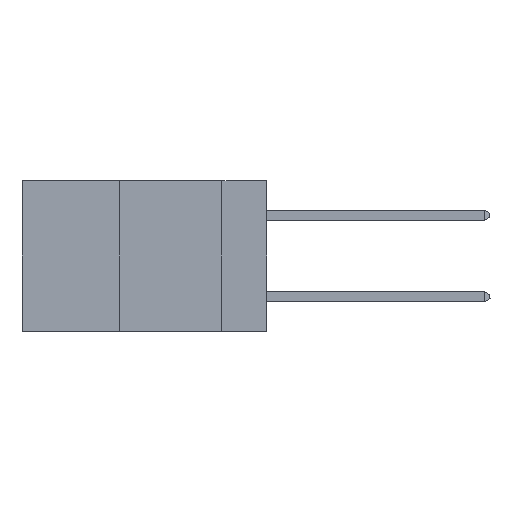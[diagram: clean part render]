
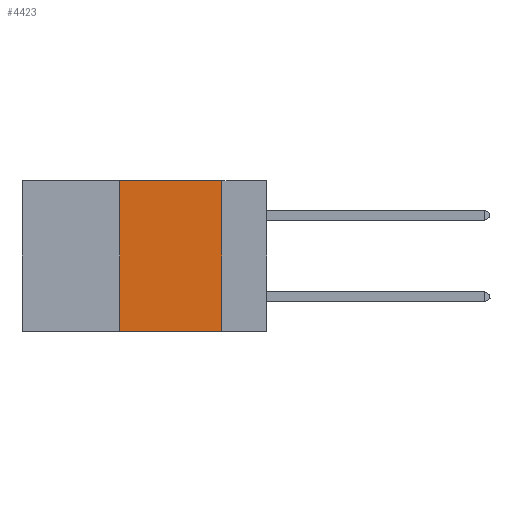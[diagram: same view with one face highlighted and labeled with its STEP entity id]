
A CAD part, left-side view. The second image highlights one B-rep face of the part: STEP entity #4423.
In plain terms, the highlighted planar face has unit normal (-1, 0, 0).
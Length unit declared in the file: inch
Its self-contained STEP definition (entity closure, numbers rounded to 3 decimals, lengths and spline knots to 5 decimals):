
#559 = CARTESIAN_POINT ( 'NONE',  ( 0., 0.36, -0.37 ) ) ;
#588 = EDGE_CURVE ( 'NONE', #12321, #1417, #3090, .T. ) ;
#690 = DIRECTION ( 'NONE',  ( 0., 0., -1. ) ) ;
#1274 = ORIENTED_EDGE ( 'NONE', *, *, #3886, .F. ) ;
#1417 = VERTEX_POINT ( 'NONE', #10688 ) ;
#1654 = VECTOR ( 'NONE', #15829, 39.37008 ) ;
#2398 = CARTESIAN_POINT ( 'NONE',  ( 0., 0.6, -0.37 ) ) ;
#2725 = ORIENTED_EDGE ( 'NONE', *, *, #12848, .F. ) ;
#2737 = VERTEX_POINT ( 'NONE', #11798 ) ;
#3090 = LINE ( 'NONE', #2398, #12622 ) ;
#3165 = ORIENTED_EDGE ( 'NONE', *, *, #588, .T. ) ;
#3886 = EDGE_CURVE ( 'NONE', #7352, #1417, #9478, .T. ) ;
#4423 = ADVANCED_FACE ( 'NONE', ( #5121 ), #16276, .F. ) ;
#5121 = FACE_OUTER_BOUND ( 'NONE', #7189, .T. ) ;
#7189 = EDGE_LOOP ( 'NONE', ( #1274, #9500, #2725, #3165 ) ) ;
#7352 = VERTEX_POINT ( 'NONE', #15607 ) ;
#7427 = LINE ( 'NONE', #10276, #13928 ) ;
#8533 = DIRECTION ( 'NONE',  ( 1., 0., 0. ) ) ;
#9025 = LINE ( 'NONE', #14522, #1654 ) ;
#9478 = LINE ( 'NONE', #13418, #15942 ) ;
#9500 = ORIENTED_EDGE ( 'NONE', *, *, #10750, .F. ) ;
#10276 = CARTESIAN_POINT ( 'NONE',  ( 0., 0.6, 0. ) ) ;
#10688 = CARTESIAN_POINT ( 'NONE',  ( 0., 0.11, -0.37 ) ) ;
#10750 = EDGE_CURVE ( 'NONE', #2737, #7352, #7427, .T. ) ;
#11566 = DIRECTION ( 'NONE',  ( 0., -1., 0. ) ) ;
#11798 = CARTESIAN_POINT ( 'NONE',  ( 0., 0.36, 0. ) ) ;
#12321 = VERTEX_POINT ( 'NONE', #559 ) ;
#12339 = CARTESIAN_POINT ( 'NONE',  ( 0., 0.6, 0. ) ) ;
#12569 = DIRECTION ( 'NONE',  ( 0., -1., 0. ) ) ;
#12622 = VECTOR ( 'NONE', #12569, 39.37008 ) ;
#12848 = EDGE_CURVE ( 'NONE', #12321, #2737, #9025, .T. ) ;
#13197 = DIRECTION ( 'NONE',  ( 0., 0., -1. ) ) ;
#13418 = CARTESIAN_POINT ( 'NONE',  ( 0., 0.11, 0. ) ) ;
#13928 = VECTOR ( 'NONE', #11566, 39.37008 ) ;
#14349 = AXIS2_PLACEMENT_3D ( 'NONE', #12339, #8533, #690 ) ;
#14522 = CARTESIAN_POINT ( 'NONE',  ( 0., 0.36, 0. ) ) ;
#15607 = CARTESIAN_POINT ( 'NONE',  ( 0., 0.11, 0. ) ) ;
#15829 = DIRECTION ( 'NONE',  ( 0., 0., 1. ) ) ;
#15942 = VECTOR ( 'NONE', #13197, 39.37008 ) ;
#16276 = PLANE ( 'NONE',  #14349 ) ;
